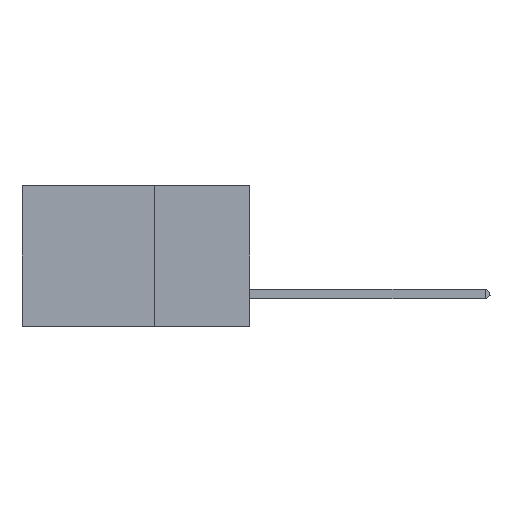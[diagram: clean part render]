
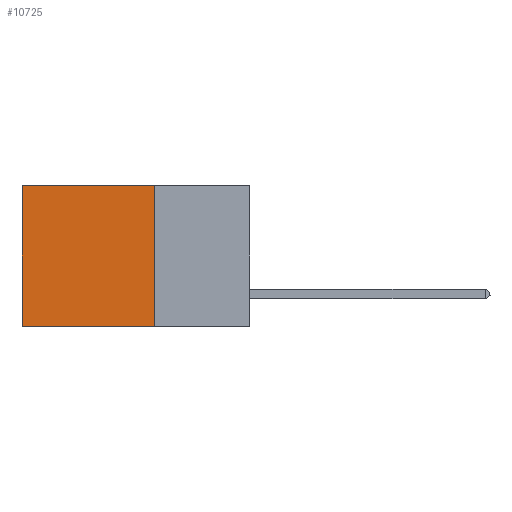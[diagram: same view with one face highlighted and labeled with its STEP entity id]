
A CAD part, left-side view. The second image highlights one B-rep face of the part: STEP entity #10725.
In plain terms, the highlighted planar face has unit normal (-1, 0, 0).
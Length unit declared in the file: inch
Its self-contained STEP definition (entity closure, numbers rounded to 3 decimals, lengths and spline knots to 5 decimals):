
#765 = ORIENTED_EDGE ( 'NONE', *, *, #15303, .T. ) ;
#1630 = DIRECTION ( 'NONE',  ( 0., 1., 0. ) ) ;
#1814 = VERTEX_POINT ( 'NONE', #24775 ) ;
#3295 = LINE ( 'NONE', #22516, #22072 ) ;
#4628 = CARTESIAN_POINT ( 'NONE',  ( 0.2875, 0.25, 0. ) ) ;
#4763 = DIRECTION ( 'NONE',  ( 0., 1., 0. ) ) ;
#4894 = VERTEX_POINT ( 'NONE', #9791 ) ;
#5551 = AXIS2_PLACEMENT_3D ( 'NONE', #7740, #20786, #27365 ) ;
#5835 = CARTESIAN_POINT ( 'NONE',  ( 0.2875, 0.25, -0.37 ) ) ;
#5992 = ORIENTED_EDGE ( 'NONE', *, *, #21753, .F. ) ;
#7255 = LINE ( 'NONE', #9511, #22100 ) ;
#7740 = CARTESIAN_POINT ( 'NONE',  ( 0.2875, 0.25, 0. ) ) ;
#7849 = VERTEX_POINT ( 'NONE', #4628 ) ;
#8491 = CARTESIAN_POINT ( 'NONE',  ( 0.2875, 0.25, -0.37 ) ) ;
#9511 = CARTESIAN_POINT ( 'NONE',  ( 0.2875, 0.6, 0. ) ) ;
#9791 = CARTESIAN_POINT ( 'NONE',  ( 0.2875, 0.6, 0. ) ) ;
#10725 = ADVANCED_FACE ( 'NONE', ( #27230 ), #12238, .F. ) ;
#11210 = ORIENTED_EDGE ( 'NONE', *, *, #12914, .F. ) ;
#12238 = PLANE ( 'NONE',  #5551 ) ;
#12914 = EDGE_CURVE ( 'NONE', #7849, #20566, #3295, .T. ) ;
#15303 = EDGE_CURVE ( 'NONE', #7849, #4894, #25667, .T. ) ;
#18196 = DIRECTION ( 'NONE',  ( 0., 0., -1. ) ) ;
#18402 = VECTOR ( 'NONE', #1630, 39.37008 ) ;
#19707 = EDGE_CURVE ( 'NONE', #4894, #1814, #7255, .T. ) ;
#20276 = DIRECTION ( 'NONE',  ( 0., 0., -1. ) ) ;
#20566 = VERTEX_POINT ( 'NONE', #8491 ) ;
#20786 = DIRECTION ( 'NONE',  ( 1., 0., 0. ) ) ;
#20853 = LINE ( 'NONE', #5835, #18402 ) ;
#21753 = EDGE_CURVE ( 'NONE', #20566, #1814, #20853, .T. ) ;
#21789 = EDGE_LOOP ( 'NONE', ( #21887, #5992, #11210, #765 ) ) ;
#21887 = ORIENTED_EDGE ( 'NONE', *, *, #19707, .T. ) ;
#22072 = VECTOR ( 'NONE', #20276, 39.37008 ) ;
#22100 = VECTOR ( 'NONE', #18196, 39.37008 ) ;
#22516 = CARTESIAN_POINT ( 'NONE',  ( 0.2875, 0.25, 0. ) ) ;
#22887 = VECTOR ( 'NONE', #4763, 39.37008 ) ;
#24775 = CARTESIAN_POINT ( 'NONE',  ( 0.2875, 0.6, -0.37 ) ) ;
#25667 = LINE ( 'NONE', #25943, #22887 ) ;
#25943 = CARTESIAN_POINT ( 'NONE',  ( 0.2875, 0.25, 0. ) ) ;
#27230 = FACE_OUTER_BOUND ( 'NONE', #21789, .T. ) ;
#27365 = DIRECTION ( 'NONE',  ( 0., 0., -1. ) ) ;
